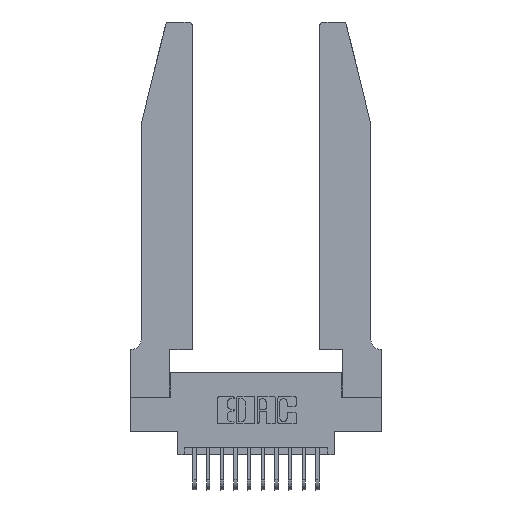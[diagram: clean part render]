
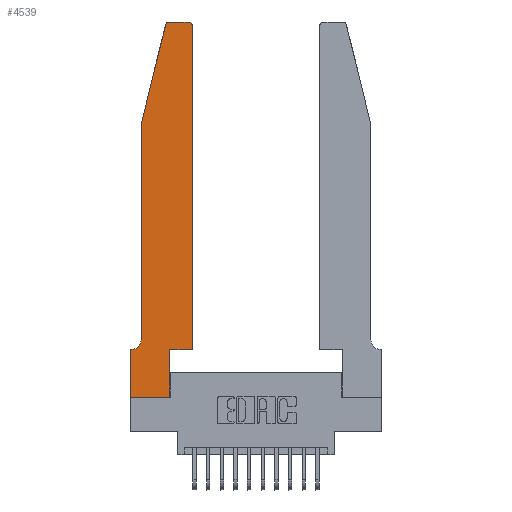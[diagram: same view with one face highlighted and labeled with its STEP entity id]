
A CAD part, top view. The second image highlights one B-rep face of the part: STEP entity #4539.
In plain terms, the highlighted planar face has unit normal (0, 0, 1).
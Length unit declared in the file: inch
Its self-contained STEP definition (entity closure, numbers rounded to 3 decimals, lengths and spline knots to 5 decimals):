
#446 = VECTOR ( 'NONE', #16184, 39.37008 ) ;
#1029 = VECTOR ( 'NONE', #8771, 39.37008 ) ;
#1198 = ORIENTED_EDGE ( 'NONE', *, *, #14913, .T. ) ;
#1200 = ORIENTED_EDGE ( 'NONE', *, *, #2764, .T. ) ;
#1273 = CARTESIAN_POINT ( 'NONE',  ( 0.4205, 2.75, 0.37 ) ) ;
#1464 = EDGE_CURVE ( 'NONE', #13400, #5342, #10446, .T. ) ;
#1493 = EDGE_CURVE ( 'NONE', #1546, #16367, #2792, .T. ) ;
#1546 = VERTEX_POINT ( 'NONE', #13127 ) ;
#1762 = CIRCLE ( 'NONE', #5315, 0.03 ) ;
#2164 = VERTEX_POINT ( 'NONE', #3254 ) ;
#2177 = DIRECTION ( 'NONE',  ( 0., 0., 1. ) ) ;
#2254 = VECTOR ( 'NONE', #3032, 39.37008 ) ;
#2517 = ORIENTED_EDGE ( 'NONE', *, *, #6547, .T. ) ;
#2764 = EDGE_CURVE ( 'NONE', #2164, #1546, #9521, .T. ) ;
#2792 = LINE ( 'NONE', #8713, #1029 ) ;
#2967 = CARTESIAN_POINT ( 'NONE',  ( 0.2865, 0., 0.37 ) ) ;
#2990 = DIRECTION ( 'NONE',  ( 0., 0., 1. ) ) ;
#3032 = DIRECTION ( 'NONE',  ( 0., 1., 0. ) ) ;
#3052 = DIRECTION ( 'NONE',  ( 1., 0., 0. ) ) ;
#3068 = CARTESIAN_POINT ( 'NONE',  ( 0.0755, 0.42, 0.37 ) ) ;
#3254 = CARTESIAN_POINT ( 'NONE',  ( 0.2865, 0.35, 0.37 ) ) ;
#3394 = CARTESIAN_POINT ( 'NONE',  ( 0.4505, 0.35, 0.37 ) ) ;
#3487 = ORIENTED_EDGE ( 'NONE', *, *, #10401, .T. ) ;
#3530 = LINE ( 'NONE', #11845, #11636 ) ;
#3685 = DIRECTION ( 'NONE',  ( 1., 0., 0. ) ) ;
#3711 = VERTEX_POINT ( 'NONE', #3887 ) ;
#3887 = CARTESIAN_POINT ( 'NONE',  ( 0., 0., 0.37 ) ) ;
#3899 = ORIENTED_EDGE ( 'NONE', *, *, #8053, .T. ) ;
#4129 = VERTEX_POINT ( 'NONE', #3068 ) ;
#4341 = EDGE_CURVE ( 'NONE', #5029, #10046, #18322, .T. ) ;
#4539 = ADVANCED_FACE ( 'NONE', ( #12831 ), #9766, .T. ) ;
#4650 = DIRECTION ( 'NONE',  ( 1., 0., 0. ) ) ;
#4840 = ORIENTED_EDGE ( 'NONE', *, *, #17401, .T. ) ;
#4844 = AXIS2_PLACEMENT_3D ( 'NONE', #16920, #2990, #3052 ) ;
#5017 = EDGE_CURVE ( 'NONE', #4129, #5029, #17609, .T. ) ;
#5029 = VERTEX_POINT ( 'NONE', #11081 ) ;
#5119 = CARTESIAN_POINT ( 'NONE',  ( 0.0755, 2., 0.37 ) ) ;
#5172 = LINE ( 'NONE', #16000, #446 ) ;
#5261 = DIRECTION ( 'NONE',  ( 0., 0., -1. ) ) ;
#5315 = AXIS2_PLACEMENT_3D ( 'NONE', #12186, #2177, #3685 ) ;
#5342 = VERTEX_POINT ( 'NONE', #10994 ) ;
#5450 = LINE ( 'NONE', #8483, #5894 ) ;
#5487 = CARTESIAN_POINT ( 'NONE',  ( 0.25487, 2.72718, 0.37 ) ) ;
#5512 = VECTOR ( 'NONE', #8838, 39.37008 ) ;
#5635 = EDGE_CURVE ( 'NONE', #7698, #12816, #5172, .T. ) ;
#5883 = AXIS2_PLACEMENT_3D ( 'NONE', #13928, #14046, #15659 ) ;
#5894 = VECTOR ( 'NONE', #14228, 39.37008 ) ;
#6298 = CARTESIAN_POINT ( 'NONE',  ( 0.4505, 2.72, 0.37 ) ) ;
#6322 = VECTOR ( 'NONE', #9236, 39.37008 ) ;
#6530 = ORIENTED_EDGE ( 'NONE', *, *, #5017, .T. ) ;
#6547 = EDGE_CURVE ( 'NONE', #16367, #13400, #1762, .T. ) ;
#6942 = CARTESIAN_POINT ( 'NONE',  ( 0.0755, 2., 0.37 ) ) ;
#7696 = ORIENTED_EDGE ( 'NONE', *, *, #9771, .T. ) ;
#7698 = VERTEX_POINT ( 'NONE', #5487 ) ;
#8053 = EDGE_CURVE ( 'NONE', #5342, #7698, #9061, .T. ) ;
#8089 = LINE ( 'NONE', #8607, #2254 ) ;
#8483 = CARTESIAN_POINT ( 'NONE',  ( 0., 0., 0.37 ) ) ;
#8607 = CARTESIAN_POINT ( 'NONE',  ( 0.2865, 0.35, 0.37 ) ) ;
#8713 = CARTESIAN_POINT ( 'NONE',  ( 0.4505, 0.35, 0.37 ) ) ;
#8771 = DIRECTION ( 'NONE',  ( 0., 1., 0. ) ) ;
#8838 = DIRECTION ( 'NONE',  ( -1., 0., 0. ) ) ;
#9061 = CIRCLE ( 'NONE', #4844, 0.03 ) ;
#9201 = DIRECTION ( 'NONE',  ( -1., 0., 0. ) ) ;
#9236 = DIRECTION ( 'NONE',  ( 0., -1., 0. ) ) ;
#9317 = ORIENTED_EDGE ( 'NONE', *, *, #4341, .T. ) ;
#9466 = AXIS2_PLACEMENT_3D ( 'NONE', #11025, #5261, #9566 ) ;
#9521 = LINE ( 'NONE', #3394, #11096 ) ;
#9566 = DIRECTION ( 'NONE',  ( -1., 0., 0. ) ) ;
#9766 = PLANE ( 'NONE',  #5883 ) ;
#9771 = EDGE_CURVE ( 'NONE', #10046, #3711, #5450, .T. ) ;
#9801 = VERTEX_POINT ( 'NONE', #2967 ) ;
#10046 = VERTEX_POINT ( 'NONE', #18315 ) ;
#10401 = EDGE_CURVE ( 'NONE', #9801, #2164, #8089, .T. ) ;
#10446 = LINE ( 'NONE', #17344, #5512 ) ;
#10867 = ORIENTED_EDGE ( 'NONE', *, *, #5635, .T. ) ;
#10994 = CARTESIAN_POINT ( 'NONE',  ( 0.284, 2.75, 0.37 ) ) ;
#11025 = CARTESIAN_POINT ( 'NONE',  ( 0.0055, 0.42, 0.37 ) ) ;
#11081 = CARTESIAN_POINT ( 'NONE',  ( 0.0055, 0.35, 0.37 ) ) ;
#11096 = VECTOR ( 'NONE', #13437, 39.37008 ) ;
#11636 = VECTOR ( 'NONE', #4650, 39.37008 ) ;
#11845 = CARTESIAN_POINT ( 'NONE',  ( 0., 0., 0.37 ) ) ;
#11855 = CARTESIAN_POINT ( 'NONE',  ( 0.0755, 0.35, 0.37 ) ) ;
#12186 = CARTESIAN_POINT ( 'NONE',  ( 0.4205, 2.72, 0.37 ) ) ;
#12404 = LINE ( 'NONE', #5119, #6322 ) ;
#12816 = VERTEX_POINT ( 'NONE', #6942 ) ;
#12831 = FACE_OUTER_BOUND ( 'NONE', #16131, .T. ) ;
#13036 = ORIENTED_EDGE ( 'NONE', *, *, #1493, .T. ) ;
#13127 = CARTESIAN_POINT ( 'NONE',  ( 0.4505, 0.35, 0.37 ) ) ;
#13400 = VERTEX_POINT ( 'NONE', #1273 ) ;
#13437 = DIRECTION ( 'NONE',  ( 1., 0., 0. ) ) ;
#13928 = CARTESIAN_POINT ( 'NONE',  ( 0., 0.35, 0.37 ) ) ;
#14046 = DIRECTION ( 'NONE',  ( 0., 0., 1. ) ) ;
#14228 = DIRECTION ( 'NONE',  ( 0., -1., 0. ) ) ;
#14434 = VECTOR ( 'NONE', #9201, 39.37008 ) ;
#14913 = EDGE_CURVE ( 'NONE', #12816, #4129, #12404, .T. ) ;
#15659 = DIRECTION ( 'NONE',  ( 1., 0., 0. ) ) ;
#16000 = CARTESIAN_POINT ( 'NONE',  ( 0.0755, 2., 0.37 ) ) ;
#16131 = EDGE_LOOP ( 'NONE', ( #18393, #3899, #10867, #1198, #6530, #9317, #7696, #4840, #3487, #1200, #13036, #2517 ) ) ;
#16184 = DIRECTION ( 'NONE',  ( -0.239, -0.971, 0. ) ) ;
#16367 = VERTEX_POINT ( 'NONE', #6298 ) ;
#16920 = CARTESIAN_POINT ( 'NONE',  ( 0.284, 2.72, 0.37 ) ) ;
#17344 = CARTESIAN_POINT ( 'NONE',  ( 0.2605, 2.75, 0.37 ) ) ;
#17401 = EDGE_CURVE ( 'NONE', #3711, #9801, #3530, .T. ) ;
#17609 = CIRCLE ( 'NONE', #9466, 0.07 ) ;
#18315 = CARTESIAN_POINT ( 'NONE',  ( 0., 0.35, 0.37 ) ) ;
#18322 = LINE ( 'NONE', #11855, #14434 ) ;
#18393 = ORIENTED_EDGE ( 'NONE', *, *, #1464, .T. ) ;
